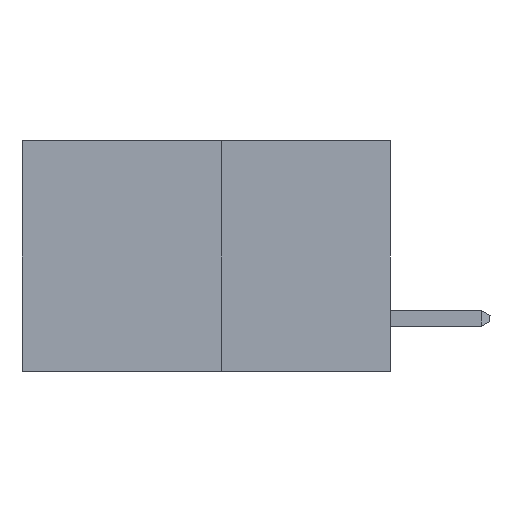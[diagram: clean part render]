
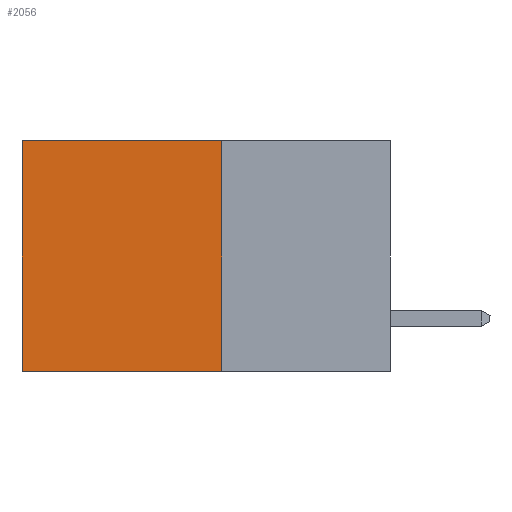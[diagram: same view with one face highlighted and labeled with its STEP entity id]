
A CAD part, left-side view. The second image highlights one B-rep face of the part: STEP entity #2056.
In plain terms, the highlighted planar face has unit normal (-1, 0, 0).
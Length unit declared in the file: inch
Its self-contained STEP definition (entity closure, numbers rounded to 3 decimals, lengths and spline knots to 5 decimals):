
#147 = VECTOR ( 'NONE', #3874, 39.37008 ) ;
#970 = DIRECTION ( 'NONE',  ( 0., 1., 0. ) ) ;
#2056 = ADVANCED_FACE ( 'NONE', ( #6718 ), #8624, .F. ) ;
#2602 = VECTOR ( 'NONE', #8845, 39.37008 ) ;
#2693 = ORIENTED_EDGE ( 'NONE', *, *, #16271, .T. ) ;
#3473 = DIRECTION ( 'NONE',  ( 1., 0., 0. ) ) ;
#3571 = AXIS2_PLACEMENT_3D ( 'NONE', #3985, #3473, #11687 ) ;
#3874 = DIRECTION ( 'NONE',  ( 0., 0., -1. ) ) ;
#3945 = LINE ( 'NONE', #15430, #14057 ) ;
#3985 = CARTESIAN_POINT ( 'NONE',  ( 0.277, 0.27, -0.37 ) ) ;
#3989 = ORIENTED_EDGE ( 'NONE', *, *, #7112, .F. ) ;
#4117 = LINE ( 'NONE', #13070, #147 ) ;
#4822 = EDGE_CURVE ( 'NONE', #12542, #6785, #9311, .T. ) ;
#6718 = FACE_OUTER_BOUND ( 'NONE', #14131, .T. ) ;
#6785 = VERTEX_POINT ( 'NONE', #13000 ) ;
#7112 = EDGE_CURVE ( 'NONE', #15621, #12542, #7781, .T. ) ;
#7346 = VECTOR ( 'NONE', #8878, 39.37008 ) ;
#7781 = LINE ( 'NONE', #8762, #7346 ) ;
#8624 = PLANE ( 'NONE',  #3571 ) ;
#8762 = CARTESIAN_POINT ( 'NONE',  ( 0.277, 0.27, -0.37 ) ) ;
#8845 = DIRECTION ( 'NONE',  ( 0., 1., 0. ) ) ;
#8878 = DIRECTION ( 'NONE',  ( 0., 0., -1. ) ) ;
#9051 = CARTESIAN_POINT ( 'NONE',  ( 0.277, 0.27, -0.37 ) ) ;
#9311 = LINE ( 'NONE', #9051, #2602 ) ;
#9836 = CARTESIAN_POINT ( 'NONE',  ( 0.277, 0.27, -0.37 ) ) ;
#11687 = DIRECTION ( 'NONE',  ( 0., 0., -1. ) ) ;
#12265 = EDGE_CURVE ( 'NONE', #16977, #6785, #4117, .T. ) ;
#12542 = VERTEX_POINT ( 'NONE', #9836 ) ;
#13000 = CARTESIAN_POINT ( 'NONE',  ( 0.277, 0.59, -0.37 ) ) ;
#13070 = CARTESIAN_POINT ( 'NONE',  ( 0.277, 0.59, -0.37 ) ) ;
#13505 = ORIENTED_EDGE ( 'NONE', *, *, #12265, .T. ) ;
#14057 = VECTOR ( 'NONE', #970, 39.37008 ) ;
#14131 = EDGE_LOOP ( 'NONE', ( #13505, #15698, #3989, #2693 ) ) ;
#15430 = CARTESIAN_POINT ( 'NONE',  ( 0.277, 0.27, 0. ) ) ;
#15433 = CARTESIAN_POINT ( 'NONE',  ( 0.277, 0.59, 0. ) ) ;
#15621 = VERTEX_POINT ( 'NONE', #16632 ) ;
#15698 = ORIENTED_EDGE ( 'NONE', *, *, #4822, .F. ) ;
#16271 = EDGE_CURVE ( 'NONE', #15621, #16977, #3945, .T. ) ;
#16632 = CARTESIAN_POINT ( 'NONE',  ( 0.277, 0.27, 0. ) ) ;
#16977 = VERTEX_POINT ( 'NONE', #15433 ) ;
